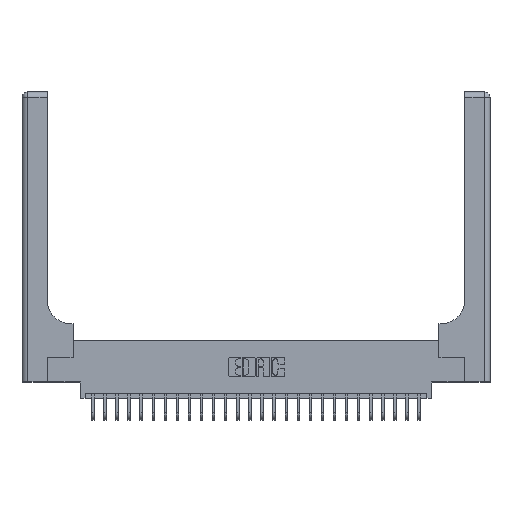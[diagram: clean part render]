
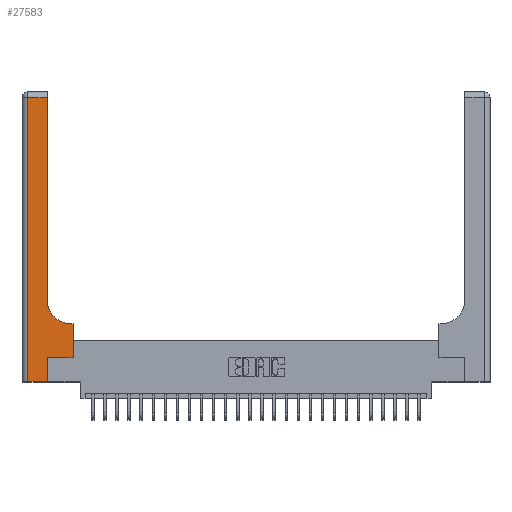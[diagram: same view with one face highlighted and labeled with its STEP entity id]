
A CAD part, top view. The second image highlights one B-rep face of the part: STEP entity #27583.
In plain terms, the highlighted planar face has unit normal (0, 0, 1).
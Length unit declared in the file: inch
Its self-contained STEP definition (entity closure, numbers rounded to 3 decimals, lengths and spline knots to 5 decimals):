
#535 = EDGE_CURVE ( 'NONE', #11965, #2794, #681, .T. ) ;
#681 = LINE ( 'NONE', #24244, #5541 ) ;
#874 = LINE ( 'NONE', #22334, #4918 ) ;
#2254 = CARTESIAN_POINT ( 'NONE',  ( 0., 3., 0.37 ) ) ;
#2279 = LINE ( 'NONE', #10579, #11285 ) ;
#2324 = EDGE_CURVE ( 'NONE', #15029, #4720, #17649, .T. ) ;
#2618 = DIRECTION ( 'NONE',  ( -1., 0., 0. ) ) ;
#2794 = VERTEX_POINT ( 'NONE', #19719 ) ;
#3107 = DIRECTION ( 'NONE',  ( 0., 1., 0. ) ) ;
#3517 = CARTESIAN_POINT ( 'NONE',  ( 0.06, 0., 0.37 ) ) ;
#3822 = ORIENTED_EDGE ( 'NONE', *, *, #2324, .T. ) ;
#3846 = VECTOR ( 'NONE', #23558, 39.37008 ) ;
#4053 = VECTOR ( 'NONE', #15541, 39.37008 ) ;
#4061 = DIRECTION ( 'NONE',  ( 0., 0., -1. ) ) ;
#4720 = VERTEX_POINT ( 'NONE', #19154 ) ;
#4918 = VECTOR ( 'NONE', #3107, 39.37008 ) ;
#5541 = VECTOR ( 'NONE', #2618, 39.37008 ) ;
#5741 = ORIENTED_EDGE ( 'NONE', *, *, #18834, .T. ) ;
#5921 = VERTEX_POINT ( 'NONE', #15102 ) ;
#6149 = VECTOR ( 'NONE', #7346, 39.37008 ) ;
#6499 = DIRECTION ( 'NONE',  ( 0., -1., 0. ) ) ;
#6978 = VERTEX_POINT ( 'NONE', #19640 ) ;
#7024 = EDGE_CURVE ( 'NONE', #4720, #5921, #17258, .T. ) ;
#7346 = DIRECTION ( 'NONE',  ( 1., 0., 0. ) ) ;
#8521 = CARTESIAN_POINT ( 'NONE',  ( 0.265, 0., 0.37 ) ) ;
#9191 = VECTOR ( 'NONE', #19424, 39.37008 ) ;
#10333 = EDGE_CURVE ( 'NONE', #24932, #6978, #21093, .T. ) ;
#10527 = DIRECTION ( 'NONE',  ( 1., 0., 0. ) ) ;
#10539 = CIRCLE ( 'NONE', #26219, 0.25 ) ;
#10579 = CARTESIAN_POINT ( 'NONE',  ( 0.06, 3., 0.37 ) ) ;
#10686 = DIRECTION ( 'NONE',  ( 0., 0., -1. ) ) ;
#10823 = DIRECTION ( 'NONE',  ( -1., 0., 0. ) ) ;
#11285 = VECTOR ( 'NONE', #6499, 39.37008 ) ;
#11574 = ORIENTED_EDGE ( 'NONE', *, *, #25897, .T. ) ;
#11965 = VERTEX_POINT ( 'NONE', #14564 ) ;
#12150 = EDGE_CURVE ( 'NONE', #6978, #27555, #19146, .T. ) ;
#12181 = ORIENTED_EDGE ( 'NONE', *, *, #535, .T. ) ;
#13092 = CARTESIAN_POINT ( 'NONE',  ( 0.26, 0.6, 0.37 ) ) ;
#14408 = EDGE_LOOP ( 'NONE', ( #27502, #12181, #11574, #3822, #16227, #5741, #24048, #19645, #18812 ) ) ;
#14564 = CARTESIAN_POINT ( 'NONE',  ( 0.26, 2.94, 0.37 ) ) ;
#14599 = CARTESIAN_POINT ( 'NONE',  ( 0.528, 0.25, 0.37 ) ) ;
#15029 = VERTEX_POINT ( 'NONE', #3517 ) ;
#15102 = CARTESIAN_POINT ( 'NONE',  ( 0.265, 0.25, 0.37 ) ) ;
#15541 = DIRECTION ( 'NONE',  ( 1., 0., 0. ) ) ;
#16227 = ORIENTED_EDGE ( 'NONE', *, *, #7024, .T. ) ;
#16496 = EDGE_CURVE ( 'NONE', #27555, #22915, #10539, .T. ) ;
#17258 = LINE ( 'NONE', #8521, #3846 ) ;
#17649 = LINE ( 'NONE', #26171, #4053 ) ;
#18812 = ORIENTED_EDGE ( 'NONE', *, *, #16496, .T. ) ;
#18834 = EDGE_CURVE ( 'NONE', #5921, #24932, #24061, .T. ) ;
#18863 = CARTESIAN_POINT ( 'NONE',  ( 0.528, 0.25, 0.37 ) ) ;
#19142 = FACE_OUTER_BOUND ( 'NONE', #14408, .T. ) ;
#19146 = LINE ( 'NONE', #13092, #9191 ) ;
#19154 = CARTESIAN_POINT ( 'NONE',  ( 0.265, 0., 0.37 ) ) ;
#19424 = DIRECTION ( 'NONE',  ( -1., 0., 0. ) ) ;
#19640 = CARTESIAN_POINT ( 'NONE',  ( 0.528, 0.6, 0.37 ) ) ;
#19645 = ORIENTED_EDGE ( 'NONE', *, *, #12150, .T. ) ;
#19719 = CARTESIAN_POINT ( 'NONE',  ( 0.06, 2.94, 0.37 ) ) ;
#21093 = LINE ( 'NONE', #18863, #23068 ) ;
#21228 = DIRECTION ( 'NONE',  ( 0., 1., 0. ) ) ;
#21495 = CARTESIAN_POINT ( 'NONE',  ( 0.51, 0.6, 0.37 ) ) ;
#21774 = PLANE ( 'NONE',  #23889 ) ;
#22020 = EDGE_CURVE ( 'NONE', #22915, #11965, #874, .T. ) ;
#22334 = CARTESIAN_POINT ( 'NONE',  ( 0.26, 3., 0.37 ) ) ;
#22915 = VERTEX_POINT ( 'NONE', #23358 ) ;
#23068 = VECTOR ( 'NONE', #21228, 39.37008 ) ;
#23304 = CARTESIAN_POINT ( 'NONE',  ( 0.51, 0.85, 0.37 ) ) ;
#23358 = CARTESIAN_POINT ( 'NONE',  ( 0.26, 0.85, 0.37 ) ) ;
#23558 = DIRECTION ( 'NONE',  ( 0., 1., 0. ) ) ;
#23889 = AXIS2_PLACEMENT_3D ( 'NONE', #2254, #10686, #10823 ) ;
#24048 = ORIENTED_EDGE ( 'NONE', *, *, #10333, .T. ) ;
#24061 = LINE ( 'NONE', #26154, #6149 ) ;
#24244 = CARTESIAN_POINT ( 'NONE',  ( 0., 2.94, 0.37 ) ) ;
#24932 = VERTEX_POINT ( 'NONE', #14599 ) ;
#25897 = EDGE_CURVE ( 'NONE', #2794, #15029, #2279, .T. ) ;
#26154 = CARTESIAN_POINT ( 'NONE',  ( 0.265, 0.25, 0.37 ) ) ;
#26171 = CARTESIAN_POINT ( 'NONE',  ( 0., 0., 0.37 ) ) ;
#26219 = AXIS2_PLACEMENT_3D ( 'NONE', #23304, #4061, #10527 ) ;
#27502 = ORIENTED_EDGE ( 'NONE', *, *, #22020, .T. ) ;
#27555 = VERTEX_POINT ( 'NONE', #21495 ) ;
#27583 = ADVANCED_FACE ( 'NONE', ( #19142 ), #21774, .F. ) ;
